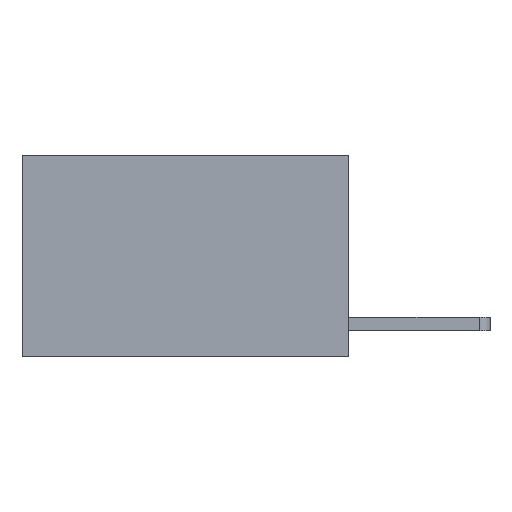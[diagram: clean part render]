
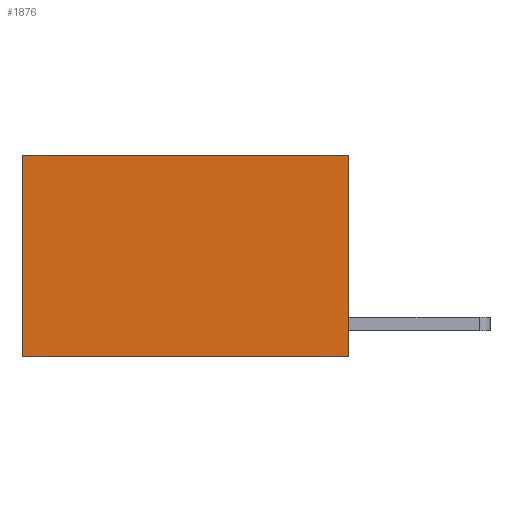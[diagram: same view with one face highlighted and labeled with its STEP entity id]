
A CAD part, left-side view. The second image highlights one B-rep face of the part: STEP entity #1876.
In plain terms, the highlighted planar face has unit normal (-1, 0, 0).
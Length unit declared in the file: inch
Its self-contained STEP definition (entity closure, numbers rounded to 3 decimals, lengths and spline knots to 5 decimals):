
#256 = DIRECTION ( 'NONE',  ( 0., 1., 0. ) ) ;
#320 = CARTESIAN_POINT ( 'NONE',  ( 0.2625, 0., 0. ) ) ;
#382 = EDGE_CURVE ( 'NONE', #6210, #9088, #6409, .T. ) ;
#1083 = DIRECTION ( 'NONE',  ( 1., 0., 0. ) ) ;
#1876 = ADVANCED_FACE ( 'NONE', ( #7722 ), #4398, .F. ) ;
#2020 = LINE ( 'NONE', #2303, #5573 ) ;
#2303 = CARTESIAN_POINT ( 'NONE',  ( 0.2625, 0., 0. ) ) ;
#2355 = EDGE_LOOP ( 'NONE', ( #6395, #7459, #5458, #4287 ) ) ;
#2511 = CARTESIAN_POINT ( 'NONE',  ( 0.2625, 0., -0.37 ) ) ;
#2520 = AXIS2_PLACEMENT_3D ( 'NONE', #6908, #1083, #3877 ) ;
#2763 = EDGE_CURVE ( 'NONE', #7643, #6210, #6285, .T. ) ;
#3235 = EDGE_CURVE ( 'NONE', #7643, #4786, #2020, .T. ) ;
#3659 = VECTOR ( 'NONE', #256, 39.37008 ) ;
#3826 = DIRECTION ( 'NONE',  ( 0., 0., -1. ) ) ;
#3877 = DIRECTION ( 'NONE',  ( 0., 0., -1. ) ) ;
#4103 = DIRECTION ( 'NONE',  ( 0., 1., 0. ) ) ;
#4154 = CARTESIAN_POINT ( 'NONE',  ( 0.2625, 0.6, 0. ) ) ;
#4287 = ORIENTED_EDGE ( 'NONE', *, *, #2763, .T. ) ;
#4398 = PLANE ( 'NONE',  #2520 ) ;
#4517 = LINE ( 'NONE', #8316, #8053 ) ;
#4786 = VERTEX_POINT ( 'NONE', #2511 ) ;
#4958 = EDGE_CURVE ( 'NONE', #4786, #9088, #4517, .T. ) ;
#5458 = ORIENTED_EDGE ( 'NONE', *, *, #3235, .F. ) ;
#5573 = VECTOR ( 'NONE', #6544, 39.37008 ) ;
#6204 = VECTOR ( 'NONE', #3826, 39.37008 ) ;
#6210 = VERTEX_POINT ( 'NONE', #4154 ) ;
#6285 = LINE ( 'NONE', #8838, #3659 ) ;
#6395 = ORIENTED_EDGE ( 'NONE', *, *, #382, .T. ) ;
#6409 = LINE ( 'NONE', #6652, #6204 ) ;
#6544 = DIRECTION ( 'NONE',  ( 0., 0., -1. ) ) ;
#6652 = CARTESIAN_POINT ( 'NONE',  ( 0.2625, 0.6, 0. ) ) ;
#6908 = CARTESIAN_POINT ( 'NONE',  ( 0.2625, 0., 0. ) ) ;
#7459 = ORIENTED_EDGE ( 'NONE', *, *, #4958, .F. ) ;
#7643 = VERTEX_POINT ( 'NONE', #320 ) ;
#7722 = FACE_OUTER_BOUND ( 'NONE', #2355, .T. ) ;
#8024 = CARTESIAN_POINT ( 'NONE',  ( 0.2625, 0.6, -0.37 ) ) ;
#8053 = VECTOR ( 'NONE', #4103, 39.37008 ) ;
#8316 = CARTESIAN_POINT ( 'NONE',  ( 0.2625, 0., -0.37 ) ) ;
#8838 = CARTESIAN_POINT ( 'NONE',  ( 0.2625, 0., 0. ) ) ;
#9088 = VERTEX_POINT ( 'NONE', #8024 ) ;
